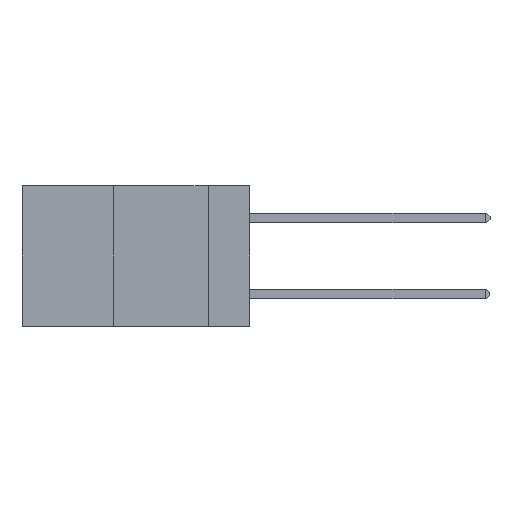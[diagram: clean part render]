
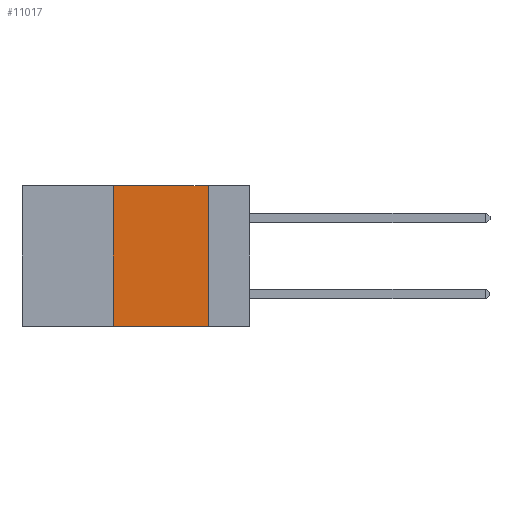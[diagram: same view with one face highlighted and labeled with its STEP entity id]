
A CAD part, left-side view. The second image highlights one B-rep face of the part: STEP entity #11017.
In plain terms, the highlighted planar face has unit normal (-1, 0, 0).
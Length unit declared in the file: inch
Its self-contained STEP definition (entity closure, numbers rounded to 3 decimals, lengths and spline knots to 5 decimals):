
#760 = PLANE ( 'NONE',  #9086 ) ;
#820 = DIRECTION ( 'NONE',  ( 0., 0., -1. ) ) ;
#936 = EDGE_CURVE ( 'NONE', #7179, #12047, #15447, .T. ) ;
#2171 = LINE ( 'NONE', #11987, #8829 ) ;
#2233 = DIRECTION ( 'NONE',  ( 0., 0., 1. ) ) ;
#2469 = LINE ( 'NONE', #7859, #15245 ) ;
#3525 = DIRECTION ( 'NONE',  ( 0., -1., 0. ) ) ;
#3563 = CARTESIAN_POINT ( 'NONE',  ( 0., 0.6, 0. ) ) ;
#3617 = VERTEX_POINT ( 'NONE', #8639 ) ;
#4553 = DIRECTION ( 'NONE',  ( 0., 0., -1. ) ) ;
#4854 = VERTEX_POINT ( 'NONE', #15040 ) ;
#5341 = ORIENTED_EDGE ( 'NONE', *, *, #13661, .F. ) ;
#5597 = EDGE_CURVE ( 'NONE', #3617, #4854, #2469, .T. ) ;
#6909 = VECTOR ( 'NONE', #2233, 39.37008 ) ;
#7179 = VERTEX_POINT ( 'NONE', #14642 ) ;
#7523 = ORIENTED_EDGE ( 'NONE', *, *, #15290, .F. ) ;
#7859 = CARTESIAN_POINT ( 'NONE',  ( 0., 0.6, -0.37 ) ) ;
#8233 = ORIENTED_EDGE ( 'NONE', *, *, #5597, .T. ) ;
#8436 = DIRECTION ( 'NONE',  ( 1., 0., 0. ) ) ;
#8639 = CARTESIAN_POINT ( 'NONE',  ( 0., 0.36, -0.37 ) ) ;
#8662 = DIRECTION ( 'NONE',  ( 0., -1., 0. ) ) ;
#8829 = VECTOR ( 'NONE', #4553, 39.37008 ) ;
#9086 = AXIS2_PLACEMENT_3D ( 'NONE', #15782, #8436, #820 ) ;
#9145 = FACE_OUTER_BOUND ( 'NONE', #9470, .T. ) ;
#9394 = CARTESIAN_POINT ( 'NONE',  ( 0., 0.11, 0. ) ) ;
#9470 = EDGE_LOOP ( 'NONE', ( #7523, #11022, #5341, #8233 ) ) ;
#11017 = ADVANCED_FACE ( 'NONE', ( #9145 ), #760, .F. ) ;
#11022 = ORIENTED_EDGE ( 'NONE', *, *, #936, .F. ) ;
#11030 = CARTESIAN_POINT ( 'NONE',  ( 0., 0.36, 0. ) ) ;
#11987 = CARTESIAN_POINT ( 'NONE',  ( 0., 0.11, 0. ) ) ;
#12047 = VERTEX_POINT ( 'NONE', #9394 ) ;
#12267 = VECTOR ( 'NONE', #8662, 39.37008 ) ;
#13534 = LINE ( 'NONE', #11030, #6909 ) ;
#13661 = EDGE_CURVE ( 'NONE', #3617, #7179, #13534, .T. ) ;
#14642 = CARTESIAN_POINT ( 'NONE',  ( 0., 0.36, 0. ) ) ;
#15040 = CARTESIAN_POINT ( 'NONE',  ( 0., 0.11, -0.37 ) ) ;
#15245 = VECTOR ( 'NONE', #3525, 39.37008 ) ;
#15290 = EDGE_CURVE ( 'NONE', #12047, #4854, #2171, .T. ) ;
#15447 = LINE ( 'NONE', #3563, #12267 ) ;
#15782 = CARTESIAN_POINT ( 'NONE',  ( 0., 0.6, 0. ) ) ;
